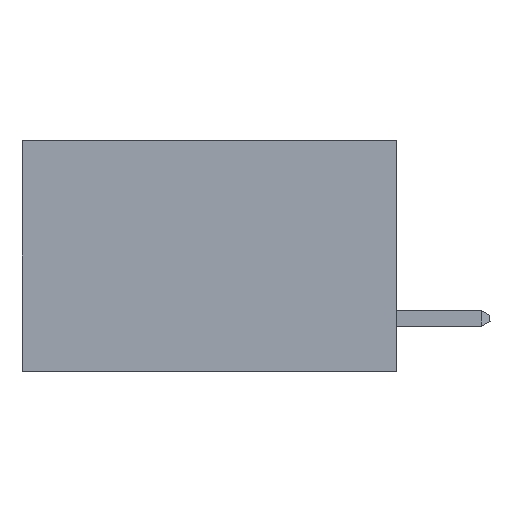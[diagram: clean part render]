
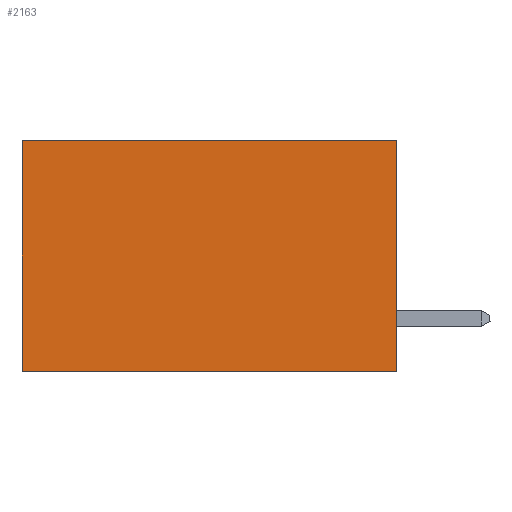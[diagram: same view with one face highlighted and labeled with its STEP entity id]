
A CAD part, left-side view. The second image highlights one B-rep face of the part: STEP entity #2163.
In plain terms, the highlighted planar face has unit normal (-1, 0, 0).
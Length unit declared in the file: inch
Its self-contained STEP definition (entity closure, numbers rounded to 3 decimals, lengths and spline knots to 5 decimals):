
#55 = PLANE ( 'NONE',  #4713 ) ;
#232 = LINE ( 'NONE', #6511, #3165 ) ;
#303 = DIRECTION ( 'NONE',  ( 0., 0., -1. ) ) ;
#822 = CARTESIAN_POINT ( 'NONE',  ( 0.298, 0.6, 0. ) ) ;
#923 = LINE ( 'NONE', #4601, #4528 ) ;
#953 = ORIENTED_EDGE ( 'NONE', *, *, #23380, .T. ) ;
#1291 = LINE ( 'NONE', #18925, #1952 ) ;
#1470 = ORIENTED_EDGE ( 'NONE', *, *, #18728, .F. ) ;
#1952 = VECTOR ( 'NONE', #20951, 39.37008 ) ;
#2163 = ADVANCED_FACE ( 'NONE', ( #3848 ), #55, .F. ) ;
#3165 = VECTOR ( 'NONE', #8636, 39.37008 ) ;
#3848 = FACE_OUTER_BOUND ( 'NONE', #17599, .T. ) ;
#4320 = EDGE_CURVE ( 'NONE', #7881, #26907, #1291, .T. ) ;
#4528 = VECTOR ( 'NONE', #303, 39.37008 ) ;
#4601 = CARTESIAN_POINT ( 'NONE',  ( 0.298, 0., 0. ) ) ;
#4713 = AXIS2_PLACEMENT_3D ( 'NONE', #14744, #25552, #18824 ) ;
#5026 = CARTESIAN_POINT ( 'NONE',  ( 0.298, 0., 0. ) ) ;
#6511 = CARTESIAN_POINT ( 'NONE',  ( 0.298, 0., 0. ) ) ;
#7589 = ORIENTED_EDGE ( 'NONE', *, *, #25669, .T. ) ;
#7881 = VERTEX_POINT ( 'NONE', #18517 ) ;
#8636 = DIRECTION ( 'NONE',  ( 0., 1., 0. ) ) ;
#9717 = VERTEX_POINT ( 'NONE', #5026 ) ;
#9764 = CARTESIAN_POINT ( 'NONE',  ( 0.298, 0.6, 0. ) ) ;
#14744 = CARTESIAN_POINT ( 'NONE',  ( 0.298, 0., 0. ) ) ;
#15283 = CARTESIAN_POINT ( 'NONE',  ( 0.298, 0.6, -0.37 ) ) ;
#15558 = LINE ( 'NONE', #822, #19184 ) ;
#17599 = EDGE_LOOP ( 'NONE', ( #7589, #21738, #1470, #953 ) ) ;
#18517 = CARTESIAN_POINT ( 'NONE',  ( 0.298, 0., -0.37 ) ) ;
#18728 = EDGE_CURVE ( 'NONE', #9717, #7881, #923, .T. ) ;
#18824 = DIRECTION ( 'NONE',  ( 0., 0., -1. ) ) ;
#18925 = CARTESIAN_POINT ( 'NONE',  ( 0.298, 0., -0.37 ) ) ;
#19184 = VECTOR ( 'NONE', #21622, 39.37008 ) ;
#20951 = DIRECTION ( 'NONE',  ( 0., 1., 0. ) ) ;
#21622 = DIRECTION ( 'NONE',  ( 0., 0., -1. ) ) ;
#21738 = ORIENTED_EDGE ( 'NONE', *, *, #4320, .F. ) ;
#23197 = VERTEX_POINT ( 'NONE', #9764 ) ;
#23380 = EDGE_CURVE ( 'NONE', #9717, #23197, #232, .T. ) ;
#25552 = DIRECTION ( 'NONE',  ( 1., 0., 0. ) ) ;
#25669 = EDGE_CURVE ( 'NONE', #23197, #26907, #15558, .T. ) ;
#26907 = VERTEX_POINT ( 'NONE', #15283 ) ;
